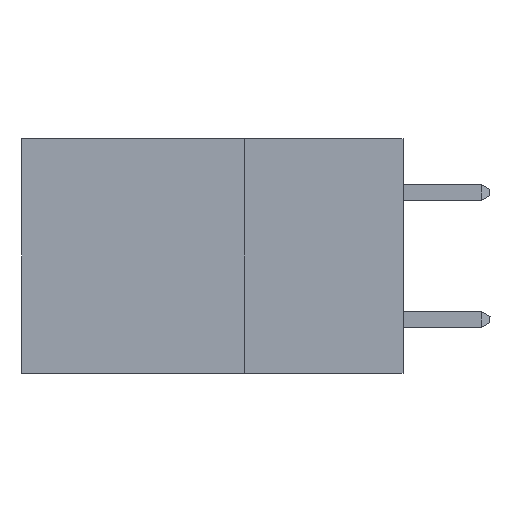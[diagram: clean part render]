
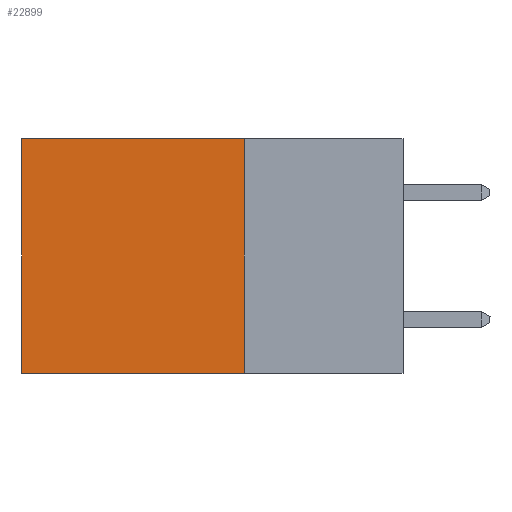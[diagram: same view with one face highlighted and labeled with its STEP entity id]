
A CAD part, left-side view. The second image highlights one B-rep face of the part: STEP entity #22899.
In plain terms, the highlighted planar face has unit normal (-1, 0, 0).
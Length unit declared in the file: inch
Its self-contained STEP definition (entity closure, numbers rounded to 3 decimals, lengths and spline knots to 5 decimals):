
#329 = ORIENTED_EDGE ( 'NONE', *, *, #11890, .F. ) ;
#555 = LINE ( 'NONE', #1898, #15065 ) ;
#866 = DIRECTION ( 'NONE',  ( 0., 0., -1. ) ) ;
#1898 = CARTESIAN_POINT ( 'NONE',  ( 0.2875, 0.25, 0. ) ) ;
#3580 = CARTESIAN_POINT ( 'NONE',  ( 0.2875, 0.25, 0. ) ) ;
#3696 = DIRECTION ( 'NONE',  ( 0., 0., -1. ) ) ;
#4028 = CARTESIAN_POINT ( 'NONE',  ( 0.2875, 0.25, 0. ) ) ;
#4885 = LINE ( 'NONE', #6452, #13530 ) ;
#5364 = VECTOR ( 'NONE', #866, 39.37008 ) ;
#5506 = DIRECTION ( 'NONE',  ( 1., 0., 0. ) ) ;
#6423 = ORIENTED_EDGE ( 'NONE', *, *, #22190, .T. ) ;
#6452 = CARTESIAN_POINT ( 'NONE',  ( 0.2875, 0.25, -0.37 ) ) ;
#7450 = CARTESIAN_POINT ( 'NONE',  ( 0.2875, 0.6, 0. ) ) ;
#8589 = EDGE_LOOP ( 'NONE', ( #6423, #16511, #329, #21808 ) ) ;
#10219 = LINE ( 'NONE', #21109, #5364 ) ;
#10593 = CARTESIAN_POINT ( 'NONE',  ( 0.2875, 0.25, 0. ) ) ;
#10842 = LINE ( 'NONE', #10593, #13721 ) ;
#11890 = EDGE_CURVE ( 'NONE', #23356, #19667, #555, .T. ) ;
#13405 = EDGE_CURVE ( 'NONE', #19667, #13680, #4885, .T. ) ;
#13530 = VECTOR ( 'NONE', #13754, 39.37008 ) ;
#13680 = VERTEX_POINT ( 'NONE', #20082 ) ;
#13721 = VECTOR ( 'NONE', #23521, 39.37008 ) ;
#13754 = DIRECTION ( 'NONE',  ( 0., 1., 0. ) ) ;
#15065 = VECTOR ( 'NONE', #16857, 39.37008 ) ;
#15073 = PLANE ( 'NONE',  #20717 ) ;
#16265 = CARTESIAN_POINT ( 'NONE',  ( 0.2875, 0.25, -0.37 ) ) ;
#16511 = ORIENTED_EDGE ( 'NONE', *, *, #13405, .F. ) ;
#16857 = DIRECTION ( 'NONE',  ( 0., 0., -1. ) ) ;
#19559 = VERTEX_POINT ( 'NONE', #7450 ) ;
#19667 = VERTEX_POINT ( 'NONE', #16265 ) ;
#19997 = FACE_OUTER_BOUND ( 'NONE', #8589, .T. ) ;
#20082 = CARTESIAN_POINT ( 'NONE',  ( 0.2875, 0.6, -0.37 ) ) ;
#20717 = AXIS2_PLACEMENT_3D ( 'NONE', #3580, #5506, #3696 ) ;
#20724 = EDGE_CURVE ( 'NONE', #23356, #19559, #10842, .T. ) ;
#21109 = CARTESIAN_POINT ( 'NONE',  ( 0.2875, 0.6, 0. ) ) ;
#21808 = ORIENTED_EDGE ( 'NONE', *, *, #20724, .T. ) ;
#22190 = EDGE_CURVE ( 'NONE', #19559, #13680, #10219, .T. ) ;
#22899 = ADVANCED_FACE ( 'NONE', ( #19997 ), #15073, .F. ) ;
#23356 = VERTEX_POINT ( 'NONE', #4028 ) ;
#23521 = DIRECTION ( 'NONE',  ( 0., 1., 0. ) ) ;
